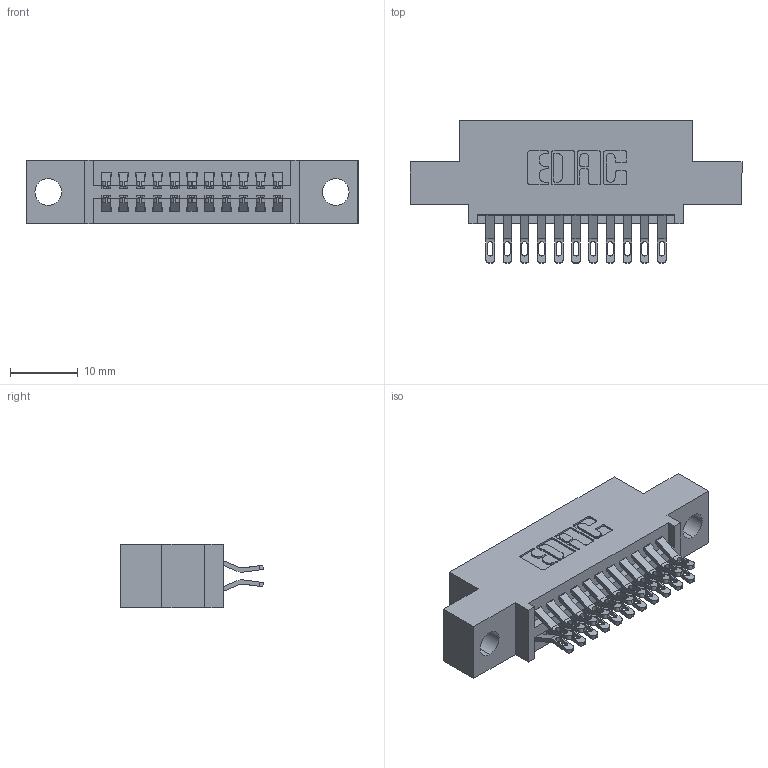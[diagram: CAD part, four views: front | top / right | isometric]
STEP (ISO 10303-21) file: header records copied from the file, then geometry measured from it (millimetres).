
FILE_DESCRIPTION (( 'STEP AP203' ), '1' );
FILE_NAME ('345-022-555-504.STEP', '2021-05-19T22:12:53', ( '' ), ( '' ), 'SwSTEP 2.0', 'SolidWorks 2020', '' );
FILE_SCHEMA (( 'CONFIG_CONTROL_DESIGN' ));
Length unit declared in the file: inch
Products named in the file (3): 345-022-555-504; 345-292-001_555 Tail; 345 Part_0.110 Offset - 0.156 Dia-TI
Assembly tree (23 placements, depth 2):
  345-022-555-504
    345 Part_0.110 Offset - 0.156 Dia-TI
    345-292-001_555 Tail  x22
Bounding box: 49.15 x 21.13 x 9.4 mm (x, y, z)
Volume: 4371.1 mm3; surface area: 6027.2 mm2
Topology: 23 solids, 23 shells, 1376 faces, 4283 edges, 2854 vertices
Faces by surface type: plane 780, cylinder 596
Entity records: 13681 total; most frequent: CARTESIAN_POINT 2364, ORIENTED_EDGE 2266, DIRECTION 2089, EDGE_CURVE 1133, LINE 937, VECTOR 937, VERTEX_POINT 754, AXIS2_PLACEMENT_3D 576
